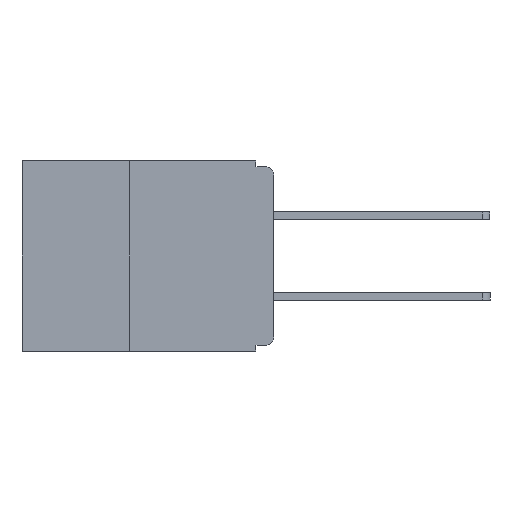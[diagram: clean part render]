
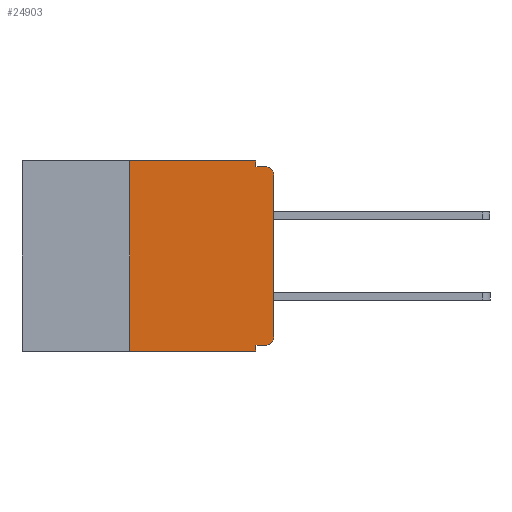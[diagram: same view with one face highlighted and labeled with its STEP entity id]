
A CAD part, left-side view. The second image highlights one B-rep face of the part: STEP entity #24903.
In plain terms, the highlighted planar face has unit normal (-1, 0, 0).
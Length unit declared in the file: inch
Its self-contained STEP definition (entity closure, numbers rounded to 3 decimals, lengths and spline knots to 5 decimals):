
#199 = ORIENTED_EDGE ( 'NONE', *, *, #6161, .F. ) ;
#1207 = AXIS2_PLACEMENT_3D ( 'NONE', #15433, #1660, #17736 ) ;
#1516 = ORIENTED_EDGE ( 'NONE', *, *, #23637, .T. ) ;
#1660 = DIRECTION ( 'NONE',  ( 1., 0., 0. ) ) ;
#1709 = EDGE_CURVE ( 'NONE', #7187, #2504, #19225, .T. ) ;
#1730 = DIRECTION ( 'NONE',  ( -1., 0., 0. ) ) ;
#2020 = CARTESIAN_POINT ( 'NONE',  ( 0., 0., 0. ) ) ;
#2192 = CARTESIAN_POINT ( 'NONE',  ( 0., 0.031, -0.01 ) ) ;
#2221 = CARTESIAN_POINT ( 'NONE',  ( 0., 0.25, -0.33 ) ) ;
#2504 = VERTEX_POINT ( 'NONE', #13733 ) ;
#2796 = VERTEX_POINT ( 'NONE', #2192 ) ;
#2951 = CARTESIAN_POINT ( 'NONE',  ( 0., 0., -0.01 ) ) ;
#3057 = DIRECTION ( 'NONE',  ( 0., -1., 0. ) ) ;
#3196 = VERTEX_POINT ( 'NONE', #11384 ) ;
#3303 = CARTESIAN_POINT ( 'NONE',  ( 0., 0.031, -0.32 ) ) ;
#3943 = EDGE_LOOP ( 'NONE', ( #1516, #11927, #21356, #199, #24221, #18807, #14805, #11155, #10691, #25946 ) ) ;
#4251 = CIRCLE ( 'NONE', #25010, 0.015 ) ;
#4497 = CARTESIAN_POINT ( 'NONE',  ( 0., 0.25, -0.33 ) ) ;
#5073 = CARTESIAN_POINT ( 'NONE',  ( 0., 0.031, -0.33 ) ) ;
#5700 = CARTESIAN_POINT ( 'NONE',  ( 0., 0.015, -0.32 ) ) ;
#5941 = VERTEX_POINT ( 'NONE', #27884 ) ;
#6161 = EDGE_CURVE ( 'NONE', #12456, #2796, #9993, .T. ) ;
#6602 = LINE ( 'NONE', #2951, #29186 ) ;
#6962 = LINE ( 'NONE', #4497, #13064 ) ;
#7182 = DIRECTION ( 'NONE',  ( 0., -1., 0. ) ) ;
#7187 = VERTEX_POINT ( 'NONE', #5700 ) ;
#8067 = LINE ( 'NONE', #15156, #13447 ) ;
#8355 = CARTESIAN_POINT ( 'NONE',  ( 0., 0.031, 0. ) ) ;
#9993 = LINE ( 'NONE', #8355, #15369 ) ;
#10691 = ORIENTED_EDGE ( 'NONE', *, *, #22185, .F. ) ;
#11155 = ORIENTED_EDGE ( 'NONE', *, *, #12299, .F. ) ;
#11384 = CARTESIAN_POINT ( 'NONE',  ( 0., 0., -0.025 ) ) ;
#11824 = AXIS2_PLACEMENT_3D ( 'NONE', #26992, #26583, #26461 ) ;
#11927 = ORIENTED_EDGE ( 'NONE', *, *, #25426, .T. ) ;
#12299 = EDGE_CURVE ( 'NONE', #16653, #17340, #18621, .T. ) ;
#12456 = VERTEX_POINT ( 'NONE', #23703 ) ;
#12471 = CARTESIAN_POINT ( 'NONE',  ( 0., 0., -0.32 ) ) ;
#12867 = LINE ( 'NONE', #2020, #24113 ) ;
#13064 = VECTOR ( 'NONE', #15912, 39.37008 ) ;
#13447 = VECTOR ( 'NONE', #21906, 39.37008 ) ;
#13733 = CARTESIAN_POINT ( 'NONE',  ( 0., 0., -0.305 ) ) ;
#13746 = VERTEX_POINT ( 'NONE', #2221 ) ;
#14805 = ORIENTED_EDGE ( 'NONE', *, *, #20707, .T. ) ;
#14812 = EDGE_CURVE ( 'NONE', #22506, #12456, #8067, .T. ) ;
#15037 = EDGE_CURVE ( 'NONE', #13746, #22506, #6962, .T. ) ;
#15156 = CARTESIAN_POINT ( 'NONE',  ( 0., 0.437, 0. ) ) ;
#15263 = EDGE_CURVE ( 'NONE', #2796, #5941, #6602, .T. ) ;
#15369 = VECTOR ( 'NONE', #17651, 39.37008 ) ;
#15433 = CARTESIAN_POINT ( 'NONE',  ( 0., 0.437, 0. ) ) ;
#15513 = CARTESIAN_POINT ( 'NONE',  ( 0., 0.015, -0.025 ) ) ;
#15912 = DIRECTION ( 'NONE',  ( 0., 0., 1. ) ) ;
#16653 = VERTEX_POINT ( 'NONE', #3303 ) ;
#17340 = VERTEX_POINT ( 'NONE', #26560 ) ;
#17651 = DIRECTION ( 'NONE',  ( 0., 0., -1. ) ) ;
#17736 = DIRECTION ( 'NONE',  ( 0., 0., -1. ) ) ;
#17814 = DIRECTION ( 'NONE',  ( 0., 0., -1. ) ) ;
#18166 = CARTESIAN_POINT ( 'NONE',  ( 0., 0.25, 0. ) ) ;
#18621 = LINE ( 'NONE', #5073, #23797 ) ;
#18630 = FACE_OUTER_BOUND ( 'NONE', #3943, .T. ) ;
#18807 = ORIENTED_EDGE ( 'NONE', *, *, #15037, .F. ) ;
#19225 = CIRCLE ( 'NONE', #11824, 0.015 ) ;
#19888 = PLANE ( 'NONE',  #1207 ) ;
#20707 = EDGE_CURVE ( 'NONE', #13746, #17340, #21135, .T. ) ;
#21135 = LINE ( 'NONE', #27415, #27755 ) ;
#21356 = ORIENTED_EDGE ( 'NONE', *, *, #15263, .F. ) ;
#21906 = DIRECTION ( 'NONE',  ( 0., -1., 0. ) ) ;
#22185 = EDGE_CURVE ( 'NONE', #7187, #16653, #28009, .T. ) ;
#22506 = VERTEX_POINT ( 'NONE', #18166 ) ;
#23208 = DIRECTION ( 'NONE',  ( 0., 0., -1. ) ) ;
#23637 = EDGE_CURVE ( 'NONE', #2504, #3196, #12867, .T. ) ;
#23694 = DIRECTION ( 'NONE',  ( 0., 1., 0. ) ) ;
#23703 = CARTESIAN_POINT ( 'NONE',  ( 0., 0.031, 0. ) ) ;
#23797 = VECTOR ( 'NONE', #23208, 39.37008 ) ;
#24113 = VECTOR ( 'NONE', #29177, 39.37008 ) ;
#24221 = ORIENTED_EDGE ( 'NONE', *, *, #14812, .F. ) ;
#24903 = ADVANCED_FACE ( 'NONE', ( #18630 ), #19888, .F. ) ;
#25010 = AXIS2_PLACEMENT_3D ( 'NONE', #15513, #1730, #17814 ) ;
#25426 = EDGE_CURVE ( 'NONE', #3196, #5941, #4251, .T. ) ;
#25946 = ORIENTED_EDGE ( 'NONE', *, *, #1709, .T. ) ;
#26461 = DIRECTION ( 'NONE',  ( 0., 0., -1. ) ) ;
#26560 = CARTESIAN_POINT ( 'NONE',  ( 0., 0.031, -0.33 ) ) ;
#26583 = DIRECTION ( 'NONE',  ( -1., 0., 0. ) ) ;
#26992 = CARTESIAN_POINT ( 'NONE',  ( 0., 0.015, -0.305 ) ) ;
#27292 = VECTOR ( 'NONE', #23694, 39.37008 ) ;
#27415 = CARTESIAN_POINT ( 'NONE',  ( 0., 0.437, -0.33 ) ) ;
#27755 = VECTOR ( 'NONE', #7182, 39.37008 ) ;
#27884 = CARTESIAN_POINT ( 'NONE',  ( 0., 0.015, -0.01 ) ) ;
#28009 = LINE ( 'NONE', #12471, #27292 ) ;
#29177 = DIRECTION ( 'NONE',  ( 0., 0., 1. ) ) ;
#29186 = VECTOR ( 'NONE', #3057, 39.37008 ) ;
